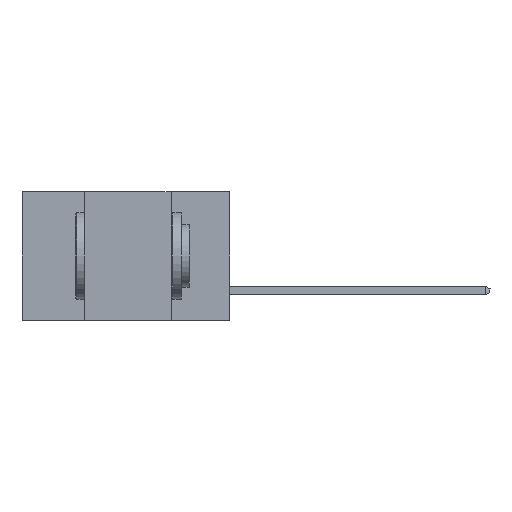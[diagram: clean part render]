
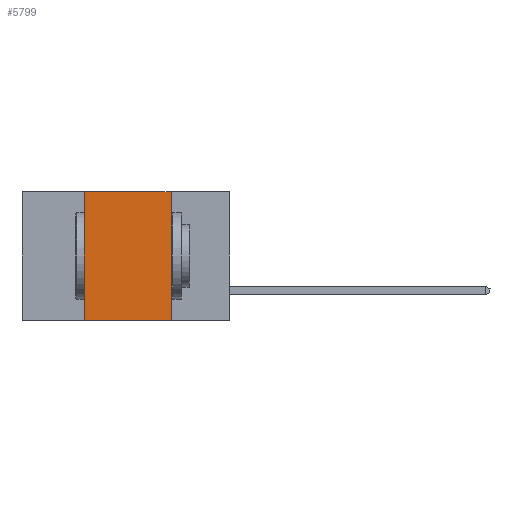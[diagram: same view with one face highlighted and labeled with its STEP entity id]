
A CAD part, left-side view. The second image highlights one B-rep face of the part: STEP entity #5799.
In plain terms, the highlighted planar face has unit normal (-1, 0, 0).
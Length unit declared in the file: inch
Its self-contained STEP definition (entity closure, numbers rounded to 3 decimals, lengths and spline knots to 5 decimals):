
#18 = VERTEX_POINT ( 'NONE', #5468 ) ;
#390 = VERTEX_POINT ( 'NONE', #8149 ) ;
#607 = VECTOR ( 'NONE', #10238, 39.37008 ) ;
#814 = ORIENTED_EDGE ( 'NONE', *, *, #8933, .F. ) ;
#923 = PLANE ( 'NONE',  #4324 ) ;
#1745 = EDGE_CURVE ( 'NONE', #18, #390, #7542, .T. ) ;
#2215 = EDGE_CURVE ( 'NONE', #2519, #390, #4896, .T. ) ;
#2519 = VERTEX_POINT ( 'NONE', #5107 ) ;
#2920 = LINE ( 'NONE', #8565, #607 ) ;
#2999 = LINE ( 'NONE', #10262, #6394 ) ;
#3560 = VECTOR ( 'NONE', #9638, 39.37008 ) ;
#4236 = DIRECTION ( 'NONE',  ( 1., 0., 0. ) ) ;
#4324 = AXIS2_PLACEMENT_3D ( 'NONE', #5089, #4236, #4343 ) ;
#4343 = DIRECTION ( 'NONE',  ( 0., 0., -1. ) ) ;
#4518 = CARTESIAN_POINT ( 'NONE',  ( 0., 0.42, 0. ) ) ;
#4701 = FACE_OUTER_BOUND ( 'NONE', #6770, .T. ) ;
#4896 = LINE ( 'NONE', #5591, #3560 ) ;
#5071 = DIRECTION ( 'NONE',  ( 0., -1., 0. ) ) ;
#5089 = CARTESIAN_POINT ( 'NONE',  ( 0., 0.6, 0. ) ) ;
#5107 = CARTESIAN_POINT ( 'NONE',  ( 0., 0.17, 0. ) ) ;
#5376 = VECTOR ( 'NONE', #5071, 39.37008 ) ;
#5468 = CARTESIAN_POINT ( 'NONE',  ( 0., 0.42, -0.37 ) ) ;
#5591 = CARTESIAN_POINT ( 'NONE',  ( 0., 0.17, -0.37 ) ) ;
#5799 = ADVANCED_FACE ( 'NONE', ( #4701 ), #923, .F. ) ;
#5871 = CARTESIAN_POINT ( 'NONE',  ( 0., 0.6, -0.37 ) ) ;
#6058 = DIRECTION ( 'NONE',  ( 0., 0., 1. ) ) ;
#6394 = VECTOR ( 'NONE', #6058, 39.37008 ) ;
#6770 = EDGE_LOOP ( 'NONE', ( #8801, #814, #8288, #8779 ) ) ;
#7542 = LINE ( 'NONE', #5871, #5376 ) ;
#7568 = VERTEX_POINT ( 'NONE', #4518 ) ;
#8064 = EDGE_CURVE ( 'NONE', #18, #7568, #2999, .T. ) ;
#8149 = CARTESIAN_POINT ( 'NONE',  ( 0., 0.17, -0.37 ) ) ;
#8288 = ORIENTED_EDGE ( 'NONE', *, *, #8064, .F. ) ;
#8565 = CARTESIAN_POINT ( 'NONE',  ( 0., 0.6, 0. ) ) ;
#8779 = ORIENTED_EDGE ( 'NONE', *, *, #1745, .T. ) ;
#8801 = ORIENTED_EDGE ( 'NONE', *, *, #2215, .F. ) ;
#8933 = EDGE_CURVE ( 'NONE', #7568, #2519, #2920, .T. ) ;
#9638 = DIRECTION ( 'NONE',  ( 0., 0., -1. ) ) ;
#10238 = DIRECTION ( 'NONE',  ( 0., -1., 0. ) ) ;
#10262 = CARTESIAN_POINT ( 'NONE',  ( 0., 0.42, -0.37 ) ) ;
